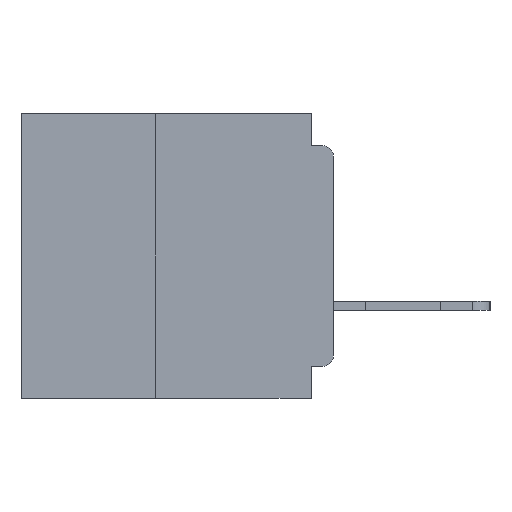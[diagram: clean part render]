
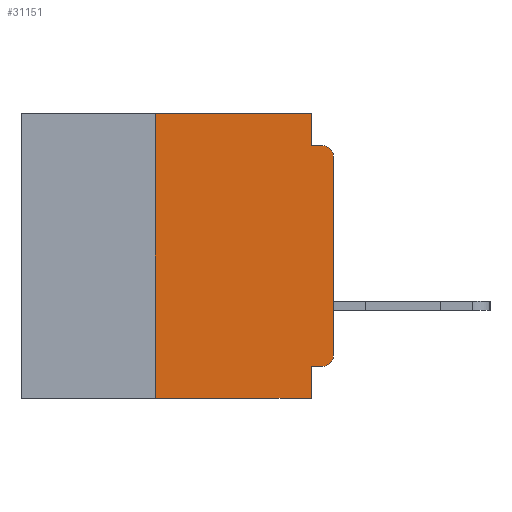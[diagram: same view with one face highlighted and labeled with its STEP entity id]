
A CAD part, left-side view. The second image highlights one B-rep face of the part: STEP entity #31151.
In plain terms, the highlighted planar face has unit normal (-1, 0, 0).
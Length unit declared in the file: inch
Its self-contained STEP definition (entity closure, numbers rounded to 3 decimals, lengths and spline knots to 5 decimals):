
#426 = CARTESIAN_POINT ( 'NONE',  ( 0., 0.031, 0. ) ) ;
#2525 = CARTESIAN_POINT ( 'NONE',  ( 0., 0.015, -0.06 ) ) ;
#3027 = ORIENTED_EDGE ( 'NONE', *, *, #41316, .F. ) ;
#3428 = DIRECTION ( 'NONE',  ( 0., 0., -1. ) ) ;
#5609 = ORIENTED_EDGE ( 'NONE', *, *, #11772, .T. ) ;
#6140 = CARTESIAN_POINT ( 'NONE',  ( 0., 0., -0.34 ) ) ;
#6280 = LINE ( 'NONE', #52579, #40168 ) ;
#6624 = EDGE_CURVE ( 'NONE', #46274, #9904, #15988, .T. ) ;
#6960 = DIRECTION ( 'NONE',  ( 0., 0., -1. ) ) ;
#7896 = VERTEX_POINT ( 'NONE', #38809 ) ;
#8011 = EDGE_CURVE ( 'NONE', #46274, #7896, #57116, .T. ) ;
#8180 = ORIENTED_EDGE ( 'NONE', *, *, #54350, .F. ) ;
#8596 = VERTEX_POINT ( 'NONE', #53326 ) ;
#8597 = CARTESIAN_POINT ( 'NONE',  ( 0., 0.015, -0.355 ) ) ;
#8739 = CARTESIAN_POINT ( 'NONE',  ( 0., 0.25, -0.4 ) ) ;
#9904 = VERTEX_POINT ( 'NONE', #6140 ) ;
#11632 = VECTOR ( 'NONE', #27513, 39.37008 ) ;
#11772 = EDGE_CURVE ( 'NONE', #9904, #43134, #22455, .T. ) ;
#15280 = ORIENTED_EDGE ( 'NONE', *, *, #32177, .T. ) ;
#15988 = CIRCLE ( 'NONE', #23505, 0.015 ) ;
#16679 = VECTOR ( 'NONE', #28562, 39.37008 ) ;
#17256 = DIRECTION ( 'NONE',  ( 0., 0., 1. ) ) ;
#17389 = CARTESIAN_POINT ( 'NONE',  ( 0., 0.437, -0.4 ) ) ;
#18211 = EDGE_CURVE ( 'NONE', #25760, #42202, #44943, .T. ) ;
#19042 = VECTOR ( 'NONE', #40269, 39.37008 ) ;
#20651 = LINE ( 'NONE', #34933, #30987 ) ;
#20794 = CARTESIAN_POINT ( 'NONE',  ( 0., 0.437, 0. ) ) ;
#22455 = LINE ( 'NONE', #46682, #44475 ) ;
#23505 = AXIS2_PLACEMENT_3D ( 'NONE', #56207, #29948, #3428 ) ;
#24087 = CARTESIAN_POINT ( 'NONE',  ( 0., 0., -0.045 ) ) ;
#24184 = ORIENTED_EDGE ( 'NONE', *, *, #6624, .T. ) ;
#25586 = DIRECTION ( 'NONE',  ( 0., 0., -1. ) ) ;
#25760 = VERTEX_POINT ( 'NONE', #8739 ) ;
#26886 = VERTEX_POINT ( 'NONE', #35160 ) ;
#27513 = DIRECTION ( 'NONE',  ( 0., 1., 0. ) ) ;
#27680 = VERTEX_POINT ( 'NONE', #36039 ) ;
#28223 = VERTEX_POINT ( 'NONE', #53838 ) ;
#28454 = LINE ( 'NONE', #24087, #16679 ) ;
#28538 = ORIENTED_EDGE ( 'NONE', *, *, #39708, .F. ) ;
#28562 = DIRECTION ( 'NONE',  ( 0., -1., 0. ) ) ;
#29665 = EDGE_LOOP ( 'NONE', ( #5609, #29879, #8180, #3027, #33251, #36990, #15280, #28538, #49936, #24184 ) ) ;
#29879 = ORIENTED_EDGE ( 'NONE', *, *, #31519, .T. ) ;
#29948 = DIRECTION ( 'NONE',  ( -1., 0., 0. ) ) ;
#30719 = DIRECTION ( 'NONE',  ( 0., 0., -1. ) ) ;
#30768 = LINE ( 'NONE', #426, #19042 ) ;
#30987 = VECTOR ( 'NONE', #39378, 39.37008 ) ;
#31151 = ADVANCED_FACE ( 'NONE', ( #43769 ), #47504, .F. ) ;
#31519 = EDGE_CURVE ( 'NONE', #43134, #8596, #45086, .T. ) ;
#32177 = EDGE_CURVE ( 'NONE', #25760, #28223, #33973, .T. ) ;
#33251 = ORIENTED_EDGE ( 'NONE', *, *, #55973, .F. ) ;
#33449 = DIRECTION ( 'NONE',  ( -1., 0., 0. ) ) ;
#33973 = LINE ( 'NONE', #17389, #44313 ) ;
#34390 = CARTESIAN_POINT ( 'NONE',  ( 0., 0.25, 0. ) ) ;
#34933 = CARTESIAN_POINT ( 'NONE',  ( 0., 0.437, 0. ) ) ;
#34973 = AXIS2_PLACEMENT_3D ( 'NONE', #2525, #33449, #6960 ) ;
#35160 = CARTESIAN_POINT ( 'NONE',  ( 0., 0.031, -0.045 ) ) ;
#36039 = CARTESIAN_POINT ( 'NONE',  ( 0., 0.031, 0. ) ) ;
#36062 = AXIS2_PLACEMENT_3D ( 'NONE', #20794, #51904, #25586 ) ;
#36990 = ORIENTED_EDGE ( 'NONE', *, *, #18211, .F. ) ;
#37820 = DIRECTION ( 'NONE',  ( 0., 0., 1. ) ) ;
#38809 = CARTESIAN_POINT ( 'NONE',  ( 0., 0.031, -0.355 ) ) ;
#39378 = DIRECTION ( 'NONE',  ( 0., -1., 0. ) ) ;
#39708 = EDGE_CURVE ( 'NONE', #7896, #28223, #6280, .T. ) ;
#40168 = VECTOR ( 'NONE', #30719, 39.37008 ) ;
#40269 = DIRECTION ( 'NONE',  ( 0., 0., -1. ) ) ;
#41316 = EDGE_CURVE ( 'NONE', #27680, #26886, #30768, .T. ) ;
#42202 = VERTEX_POINT ( 'NONE', #34390 ) ;
#43134 = VERTEX_POINT ( 'NONE', #49633 ) ;
#43651 = CARTESIAN_POINT ( 'NONE',  ( 0., 0.25, -0.4 ) ) ;
#43769 = FACE_OUTER_BOUND ( 'NONE', #29665, .T. ) ;
#43791 = DIRECTION ( 'NONE',  ( 0., -1., 0. ) ) ;
#44313 = VECTOR ( 'NONE', #43791, 39.37008 ) ;
#44475 = VECTOR ( 'NONE', #37820, 39.37008 ) ;
#44943 = LINE ( 'NONE', #43651, #56572 ) ;
#45086 = CIRCLE ( 'NONE', #34973, 0.015 ) ;
#46274 = VERTEX_POINT ( 'NONE', #8597 ) ;
#46682 = CARTESIAN_POINT ( 'NONE',  ( 0., 0., 0. ) ) ;
#47504 = PLANE ( 'NONE',  #36062 ) ;
#49633 = CARTESIAN_POINT ( 'NONE',  ( 0., 0., -0.06 ) ) ;
#49936 = ORIENTED_EDGE ( 'NONE', *, *, #8011, .F. ) ;
#51904 = DIRECTION ( 'NONE',  ( 1., 0., 0. ) ) ;
#52579 = CARTESIAN_POINT ( 'NONE',  ( 0., 0.031, -0.4 ) ) ;
#53326 = CARTESIAN_POINT ( 'NONE',  ( 0., 0.015, -0.045 ) ) ;
#53778 = CARTESIAN_POINT ( 'NONE',  ( 0., 0., -0.355 ) ) ;
#53838 = CARTESIAN_POINT ( 'NONE',  ( 0., 0.031, -0.4 ) ) ;
#54350 = EDGE_CURVE ( 'NONE', #26886, #8596, #28454, .T. ) ;
#55973 = EDGE_CURVE ( 'NONE', #42202, #27680, #20651, .T. ) ;
#56207 = CARTESIAN_POINT ( 'NONE',  ( 0., 0.015, -0.34 ) ) ;
#56572 = VECTOR ( 'NONE', #17256, 39.37008 ) ;
#57116 = LINE ( 'NONE', #53778, #11632 ) ;
